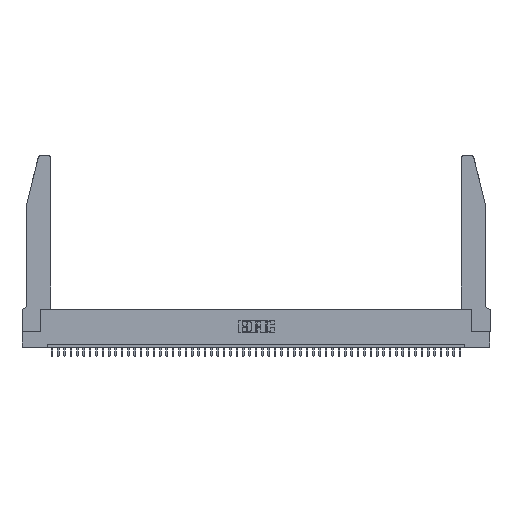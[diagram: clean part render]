
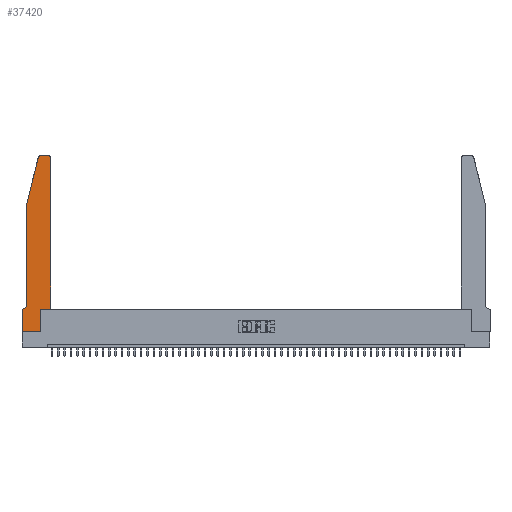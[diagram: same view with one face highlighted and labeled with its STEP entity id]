
A CAD part, top view. The second image highlights one B-rep face of the part: STEP entity #37420.
In plain terms, the highlighted planar face has unit normal (0, 0, 1).
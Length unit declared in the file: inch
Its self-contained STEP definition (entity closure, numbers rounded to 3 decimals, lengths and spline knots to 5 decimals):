
#76 = VECTOR ( 'NONE', #13676, 39.37008 ) ;
#1404 = VERTEX_POINT ( 'NONE', #27427 ) ;
#1957 = DIRECTION ( 'NONE',  ( -1., 0., 0. ) ) ;
#3254 = VERTEX_POINT ( 'NONE', #12134 ) ;
#4528 = VERTEX_POINT ( 'NONE', #49429 ) ;
#5149 = CARTESIAN_POINT ( 'NONE',  ( 0.4205, 2.75, 0.37 ) ) ;
#5732 = CARTESIAN_POINT ( 'NONE',  ( 0., 0.35, 0.37 ) ) ;
#6530 = DIRECTION ( 'NONE',  ( 0., 0., 1. ) ) ;
#6648 = DIRECTION ( 'NONE',  ( -1., 0., 0. ) ) ;
#6651 = LINE ( 'NONE', #35954, #10893 ) ;
#6657 = EDGE_CURVE ( 'NONE', #4528, #33588, #47189, .T. ) ;
#6854 = DIRECTION ( 'NONE',  ( 0., 0., 1. ) ) ;
#7240 = EDGE_CURVE ( 'NONE', #34527, #10993, #43460, .T. ) ;
#7293 = LINE ( 'NONE', #38998, #37848 ) ;
#7327 = EDGE_CURVE ( 'NONE', #40599, #19762, #8590, .T. ) ;
#8447 = CARTESIAN_POINT ( 'NONE',  ( 0.4505, 2.72, 0.37 ) ) ;
#8530 = CARTESIAN_POINT ( 'NONE',  ( 0., 0., 0.37 ) ) ;
#8590 = CIRCLE ( 'NONE', #47556, 0.03 ) ;
#9595 = CARTESIAN_POINT ( 'NONE',  ( 0.0755, 0.35, 0.37 ) ) ;
#9813 = DIRECTION ( 'NONE',  ( 0., 0., 1. ) ) ;
#10428 = LINE ( 'NONE', #48214, #76 ) ;
#10893 = VECTOR ( 'NONE', #11491, 39.37008 ) ;
#10993 = VERTEX_POINT ( 'NONE', #8447 ) ;
#11491 = DIRECTION ( 'NONE',  ( -0.239, -0.971, 0. ) ) ;
#11611 = CARTESIAN_POINT ( 'NONE',  ( 0., 0.35, 0.37 ) ) ;
#12134 = CARTESIAN_POINT ( 'NONE',  ( 0.0755, 0.42, 0.37 ) ) ;
#13027 = ORIENTED_EDGE ( 'NONE', *, *, #25447, .T. ) ;
#13040 = EDGE_CURVE ( 'NONE', #26777, #4528, #19460, .T. ) ;
#13087 = CARTESIAN_POINT ( 'NONE',  ( 0.4505, 0.35, 0.37 ) ) ;
#13348 = AXIS2_PLACEMENT_3D ( 'NONE', #42051, #6854, #34174 ) ;
#13676 = DIRECTION ( 'NONE',  ( 1., 0., 0. ) ) ;
#13942 = VERTEX_POINT ( 'NONE', #11611 ) ;
#14100 = ORIENTED_EDGE ( 'NONE', *, *, #13040, .T. ) ;
#14803 = DIRECTION ( 'NONE',  ( 0., 0., -1. ) ) ;
#15217 = VECTOR ( 'NONE', #23084, 39.37008 ) ;
#15398 = ORIENTED_EDGE ( 'NONE', *, *, #28059, .T. ) ;
#15669 = ORIENTED_EDGE ( 'NONE', *, *, #7327, .T. ) ;
#16554 = VECTOR ( 'NONE', #16623, 39.37008 ) ;
#16623 = DIRECTION ( 'NONE',  ( 0., -1., 0. ) ) ;
#16700 = CARTESIAN_POINT ( 'NONE',  ( 0.4505, 0.35, 0.37 ) ) ;
#16792 = DIRECTION ( 'NONE',  ( 0., -1., 0. ) ) ;
#17865 = VECTOR ( 'NONE', #25189, 39.37008 ) ;
#18218 = EDGE_CURVE ( 'NONE', #33588, #34527, #10428, .T. ) ;
#19459 = DIRECTION ( 'NONE',  ( -1., 0., 0. ) ) ;
#19460 = LINE ( 'NONE', #46511, #15217 ) ;
#19762 = VERTEX_POINT ( 'NONE', #31122 ) ;
#21820 = DIRECTION ( 'NONE',  ( 0., 1., 0. ) ) ;
#22099 = ORIENTED_EDGE ( 'NONE', *, *, #7240, .T. ) ;
#23084 = DIRECTION ( 'NONE',  ( 1., 0., 0. ) ) ;
#23272 = DIRECTION ( 'NONE',  ( 1., 0., 0. ) ) ;
#25189 = DIRECTION ( 'NONE',  ( 0., 1., 0. ) ) ;
#25447 = EDGE_CURVE ( 'NONE', #1404, #13942, #49904, .T. ) ;
#26308 = CARTESIAN_POINT ( 'NONE',  ( 0.284, 2.72, 0.37 ) ) ;
#26607 = ORIENTED_EDGE ( 'NONE', *, *, #18218, .T. ) ;
#26665 = ORIENTED_EDGE ( 'NONE', *, *, #6657, .T. ) ;
#26777 = VERTEX_POINT ( 'NONE', #8530 ) ;
#26918 = ORIENTED_EDGE ( 'NONE', *, *, #45616, .T. ) ;
#27427 = CARTESIAN_POINT ( 'NONE',  ( 0.0055, 0.35, 0.37 ) ) ;
#28059 = EDGE_CURVE ( 'NONE', #3254, #1404, #41169, .T. ) ;
#28702 = CARTESIAN_POINT ( 'NONE',  ( 0.0755, 2., 0.37 ) ) ;
#29601 = EDGE_CURVE ( 'NONE', #10993, #47644, #42199, .T. ) ;
#30260 = DIRECTION ( 'NONE',  ( 1., 0., 0. ) ) ;
#31062 = AXIS2_PLACEMENT_3D ( 'NONE', #34295, #14803, #6648 ) ;
#31122 = CARTESIAN_POINT ( 'NONE',  ( 0.25487, 2.72718, 0.37 ) ) ;
#32506 = VECTOR ( 'NONE', #16792, 39.37008 ) ;
#33137 = ORIENTED_EDGE ( 'NONE', *, *, #47466, .T. ) ;
#33588 = VERTEX_POINT ( 'NONE', #41195 ) ;
#34174 = DIRECTION ( 'NONE',  ( 1., 0., 0. ) ) ;
#34295 = CARTESIAN_POINT ( 'NONE',  ( 0.0055, 0.42, 0.37 ) ) ;
#34527 = VERTEX_POINT ( 'NONE', #16700 ) ;
#35954 = CARTESIAN_POINT ( 'NONE',  ( 0.0755, 2., 0.37 ) ) ;
#37370 = CARTESIAN_POINT ( 'NONE',  ( 0.2865, 0.35, 0.37 ) ) ;
#37388 = LINE ( 'NONE', #48233, #16554 ) ;
#37420 = ADVANCED_FACE ( 'NONE', ( #45944 ), #44390, .T. ) ;
#37848 = VECTOR ( 'NONE', #19459, 39.37008 ) ;
#38121 = ORIENTED_EDGE ( 'NONE', *, *, #29601, .T. ) ;
#38998 = CARTESIAN_POINT ( 'NONE',  ( 0.2605, 2.75, 0.37 ) ) ;
#39266 = LINE ( 'NONE', #40772, #32506 ) ;
#39892 = EDGE_CURVE ( 'NONE', #19762, #43429, #6651, .T. ) ;
#40599 = VERTEX_POINT ( 'NONE', #50158 ) ;
#40772 = CARTESIAN_POINT ( 'NONE',  ( 0.0755, 2., 0.37 ) ) ;
#41047 = VECTOR ( 'NONE', #21820, 39.37008 ) ;
#41139 = EDGE_LOOP ( 'NONE', ( #33137, #15669, #49324, #26918, #15398, #13027, #44692, #14100, #26665, #26607, #22099, #38121 ) ) ;
#41169 = CIRCLE ( 'NONE', #31062, 0.07 ) ;
#41195 = CARTESIAN_POINT ( 'NONE',  ( 0.2865, 0.35, 0.37 ) ) ;
#42051 = CARTESIAN_POINT ( 'NONE',  ( 0.4205, 2.72, 0.37 ) ) ;
#42199 = CIRCLE ( 'NONE', #13348, 0.03 ) ;
#43113 = AXIS2_PLACEMENT_3D ( 'NONE', #5732, #9813, #23272 ) ;
#43429 = VERTEX_POINT ( 'NONE', #28702 ) ;
#43460 = LINE ( 'NONE', #13087, #41047 ) ;
#44390 = PLANE ( 'NONE',  #43113 ) ;
#44692 = ORIENTED_EDGE ( 'NONE', *, *, #45607, .T. ) ;
#45607 = EDGE_CURVE ( 'NONE', #13942, #26777, #37388, .T. ) ;
#45616 = EDGE_CURVE ( 'NONE', #43429, #3254, #39266, .T. ) ;
#45944 = FACE_OUTER_BOUND ( 'NONE', #41139, .T. ) ;
#46511 = CARTESIAN_POINT ( 'NONE',  ( 0., 0., 0.37 ) ) ;
#47189 = LINE ( 'NONE', #37370, #17865 ) ;
#47446 = VECTOR ( 'NONE', #1957, 39.37008 ) ;
#47466 = EDGE_CURVE ( 'NONE', #47644, #40599, #7293, .T. ) ;
#47556 = AXIS2_PLACEMENT_3D ( 'NONE', #26308, #6530, #30260 ) ;
#47644 = VERTEX_POINT ( 'NONE', #5149 ) ;
#48214 = CARTESIAN_POINT ( 'NONE',  ( 0.4505, 0.35, 0.37 ) ) ;
#48233 = CARTESIAN_POINT ( 'NONE',  ( 0., 0., 0.37 ) ) ;
#49324 = ORIENTED_EDGE ( 'NONE', *, *, #39892, .T. ) ;
#49429 = CARTESIAN_POINT ( 'NONE',  ( 0.2865, 0., 0.37 ) ) ;
#49904 = LINE ( 'NONE', #9595, #47446 ) ;
#50158 = CARTESIAN_POINT ( 'NONE',  ( 0.284, 2.75, 0.37 ) ) ;
